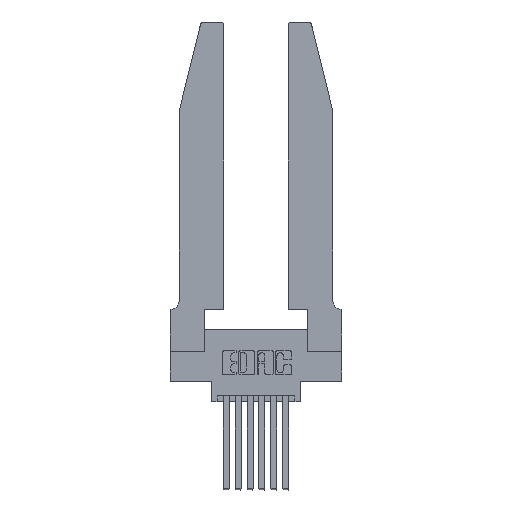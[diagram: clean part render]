
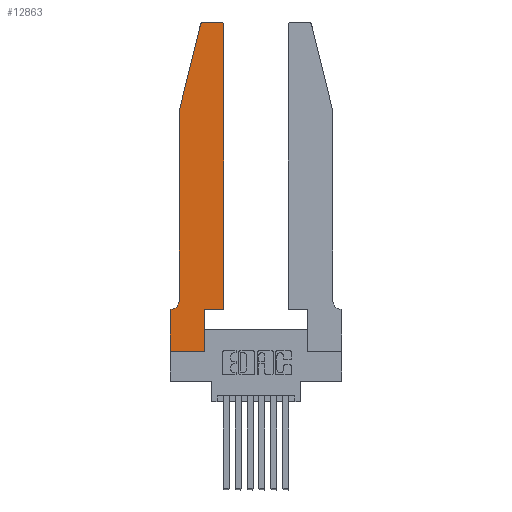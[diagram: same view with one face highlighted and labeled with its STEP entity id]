
A CAD part, top view. The second image highlights one B-rep face of the part: STEP entity #12863.
In plain terms, the highlighted planar face has unit normal (0, 0, 1).
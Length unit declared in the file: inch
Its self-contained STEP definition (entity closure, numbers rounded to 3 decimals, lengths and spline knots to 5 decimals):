
#48 = DIRECTION ( 'NONE',  ( 0., 0., -1. ) ) ;
#102 = EDGE_CURVE ( 'NONE', #6699, #5220, #8857, .T. ) ;
#254 = DIRECTION ( 'NONE',  ( -1., 0., 0. ) ) ;
#436 = CARTESIAN_POINT ( 'NONE',  ( 0.4505, 0.35, 0.37 ) ) ;
#438 = VERTEX_POINT ( 'NONE', #4271 ) ;
#738 = EDGE_CURVE ( 'NONE', #9904, #9784, #1970, .T. ) ;
#946 = LINE ( 'NONE', #7769, #11958 ) ;
#1117 = CARTESIAN_POINT ( 'NONE',  ( 0.2605, 2.75, 0.37 ) ) ;
#1137 = EDGE_CURVE ( 'NONE', #9796, #3739, #946, .T. ) ;
#1267 = EDGE_CURVE ( 'NONE', #11987, #6699, #13153, .T. ) ;
#1388 = DIRECTION ( 'NONE',  ( -0.239, -0.971, 0. ) ) ;
#1421 = CARTESIAN_POINT ( 'NONE',  ( 0.4505, 0.35, 0.37 ) ) ;
#1868 = CARTESIAN_POINT ( 'NONE',  ( 0.4205, 2.75, 0.37 ) ) ;
#1921 = ORIENTED_EDGE ( 'NONE', *, *, #8538, .T. ) ;
#1970 = LINE ( 'NONE', #13035, #2311 ) ;
#2106 = VECTOR ( 'NONE', #3798, 39.37008 ) ;
#2199 = CARTESIAN_POINT ( 'NONE',  ( 0., 0., 0.37 ) ) ;
#2261 = ORIENTED_EDGE ( 'NONE', *, *, #11199, .T. ) ;
#2276 = DIRECTION ( 'NONE',  ( 0., -1., 0. ) ) ;
#2311 = VECTOR ( 'NONE', #13481, 39.37008 ) ;
#2406 = CARTESIAN_POINT ( 'NONE',  ( 0.2865, 0.35, 0.37 ) ) ;
#2538 = DIRECTION ( 'NONE',  ( 0., 1., 0. ) ) ;
#2598 = ORIENTED_EDGE ( 'NONE', *, *, #102, .T. ) ;
#2676 = EDGE_CURVE ( 'NONE', #9784, #9796, #11205, .T. ) ;
#2685 = PLANE ( 'NONE',  #3097 ) ;
#2730 = DIRECTION ( 'NONE',  ( 0., 0., 1. ) ) ;
#3025 = VECTOR ( 'NONE', #2276, 39.37008 ) ;
#3097 = AXIS2_PLACEMENT_3D ( 'NONE', #13633, #12588, #5986 ) ;
#3138 = AXIS2_PLACEMENT_3D ( 'NONE', #6673, #48, #7772 ) ;
#3648 = EDGE_CURVE ( 'NONE', #5220, #11463, #9231, .T. ) ;
#3739 = VERTEX_POINT ( 'NONE', #2406 ) ;
#3798 = DIRECTION ( 'NONE',  ( 1., 0., 0. ) ) ;
#3972 = CARTESIAN_POINT ( 'NONE',  ( 0.4505, 2.72, 0.37 ) ) ;
#4059 = VERTEX_POINT ( 'NONE', #1868 ) ;
#4271 = CARTESIAN_POINT ( 'NONE',  ( 0.4505, 0.35, 0.37 ) ) ;
#4356 = ORIENTED_EDGE ( 'NONE', *, *, #7726, .T. ) ;
#4472 = DIRECTION ( 'NONE',  ( -1., 0., 0. ) ) ;
#4856 = CIRCLE ( 'NONE', #12831, 0.03 ) ;
#5187 = ORIENTED_EDGE ( 'NONE', *, *, #1267, .T. ) ;
#5220 = VERTEX_POINT ( 'NONE', #11902 ) ;
#5974 = CARTESIAN_POINT ( 'NONE',  ( 0.0755, 2., 0.37 ) ) ;
#5986 = DIRECTION ( 'NONE',  ( 1., 0., 0. ) ) ;
#6177 = EDGE_CURVE ( 'NONE', #11463, #9904, #12801, .T. ) ;
#6208 = ORIENTED_EDGE ( 'NONE', *, *, #738, .T. ) ;
#6221 = LINE ( 'NONE', #436, #9134 ) ;
#6491 = LINE ( 'NONE', #1421, #8011 ) ;
#6493 = CARTESIAN_POINT ( 'NONE',  ( 0.4205, 2.72, 0.37 ) ) ;
#6509 = CARTESIAN_POINT ( 'NONE',  ( 0.25487, 2.72718, 0.37 ) ) ;
#6673 = CARTESIAN_POINT ( 'NONE',  ( 0.0055, 0.42, 0.37 ) ) ;
#6699 = VERTEX_POINT ( 'NONE', #12261 ) ;
#7239 = ORIENTED_EDGE ( 'NONE', *, *, #13641, .T. ) ;
#7595 = ORIENTED_EDGE ( 'NONE', *, *, #10798, .T. ) ;
#7599 = DIRECTION ( 'NONE',  ( 1., 0., 0. ) ) ;
#7726 = EDGE_CURVE ( 'NONE', #3739, #438, #6221, .T. ) ;
#7769 = CARTESIAN_POINT ( 'NONE',  ( 0.2865, 0.35, 0.37 ) ) ;
#7772 = DIRECTION ( 'NONE',  ( -1., 0., 0. ) ) ;
#8011 = VECTOR ( 'NONE', #2538, 39.37008 ) ;
#8085 = DIRECTION ( 'NONE',  ( 1., 0., 0. ) ) ;
#8538 = EDGE_CURVE ( 'NONE', #4059, #13608, #13748, .T. ) ;
#8789 = ORIENTED_EDGE ( 'NONE', *, *, #3648, .T. ) ;
#8801 = EDGE_LOOP ( 'NONE', ( #1921, #2261, #5187, #2598, #8789, #11717, #6208, #12076, #9474, #4356, #7239, #7595 ) ) ;
#8857 = LINE ( 'NONE', #10115, #3025 ) ;
#9134 = VECTOR ( 'NONE', #8085, 39.37008 ) ;
#9231 = CIRCLE ( 'NONE', #3138, 0.07 ) ;
#9243 = CARTESIAN_POINT ( 'NONE',  ( 0., 0., 0.37 ) ) ;
#9316 = CIRCLE ( 'NONE', #10892, 0.03 ) ;
#9317 = CARTESIAN_POINT ( 'NONE',  ( 0.284, 2.72, 0.37 ) ) ;
#9474 = ORIENTED_EDGE ( 'NONE', *, *, #1137, .T. ) ;
#9784 = VERTEX_POINT ( 'NONE', #2199 ) ;
#9796 = VERTEX_POINT ( 'NONE', #13200 ) ;
#9904 = VERTEX_POINT ( 'NONE', #12423 ) ;
#10115 = CARTESIAN_POINT ( 'NONE',  ( 0.0755, 2., 0.37 ) ) ;
#10131 = DIRECTION ( 'NONE',  ( 0., 1., 0. ) ) ;
#10188 = CARTESIAN_POINT ( 'NONE',  ( 0.0755, 0.35, 0.37 ) ) ;
#10222 = VECTOR ( 'NONE', #1388, 39.37008 ) ;
#10420 = DIRECTION ( 'NONE',  ( 1., 0., 0. ) ) ;
#10798 = EDGE_CURVE ( 'NONE', #13217, #4059, #9316, .T. ) ;
#10841 = VECTOR ( 'NONE', #4472, 39.37008 ) ;
#10892 = AXIS2_PLACEMENT_3D ( 'NONE', #6493, #14167, #7599 ) ;
#11151 = FACE_OUTER_BOUND ( 'NONE', #8801, .T. ) ;
#11199 = EDGE_CURVE ( 'NONE', #13608, #11987, #4856, .T. ) ;
#11205 = LINE ( 'NONE', #9243, #2106 ) ;
#11463 = VERTEX_POINT ( 'NONE', #14240 ) ;
#11717 = ORIENTED_EDGE ( 'NONE', *, *, #6177, .T. ) ;
#11902 = CARTESIAN_POINT ( 'NONE',  ( 0.0755, 0.42, 0.37 ) ) ;
#11958 = VECTOR ( 'NONE', #10131, 39.37008 ) ;
#11987 = VERTEX_POINT ( 'NONE', #6509 ) ;
#12076 = ORIENTED_EDGE ( 'NONE', *, *, #2676, .T. ) ;
#12261 = CARTESIAN_POINT ( 'NONE',  ( 0.0755, 2., 0.37 ) ) ;
#12423 = CARTESIAN_POINT ( 'NONE',  ( 0., 0.35, 0.37 ) ) ;
#12460 = VECTOR ( 'NONE', #254, 39.37008 ) ;
#12588 = DIRECTION ( 'NONE',  ( 0., 0., 1. ) ) ;
#12801 = LINE ( 'NONE', #10188, #12460 ) ;
#12831 = AXIS2_PLACEMENT_3D ( 'NONE', #9317, #2730, #10420 ) ;
#12863 = ADVANCED_FACE ( 'NONE', ( #11151 ), #2685, .T. ) ;
#13035 = CARTESIAN_POINT ( 'NONE',  ( 0., 0., 0.37 ) ) ;
#13153 = LINE ( 'NONE', #5974, #10222 ) ;
#13200 = CARTESIAN_POINT ( 'NONE',  ( 0.2865, 0., 0.37 ) ) ;
#13217 = VERTEX_POINT ( 'NONE', #3972 ) ;
#13393 = CARTESIAN_POINT ( 'NONE',  ( 0.284, 2.75, 0.37 ) ) ;
#13481 = DIRECTION ( 'NONE',  ( 0., -1., 0. ) ) ;
#13608 = VERTEX_POINT ( 'NONE', #13393 ) ;
#13633 = CARTESIAN_POINT ( 'NONE',  ( 0., 0.35, 0.37 ) ) ;
#13641 = EDGE_CURVE ( 'NONE', #438, #13217, #6491, .T. ) ;
#13748 = LINE ( 'NONE', #1117, #10841 ) ;
#14167 = DIRECTION ( 'NONE',  ( 0., 0., 1. ) ) ;
#14240 = CARTESIAN_POINT ( 'NONE',  ( 0.0055, 0.35, 0.37 ) ) ;
